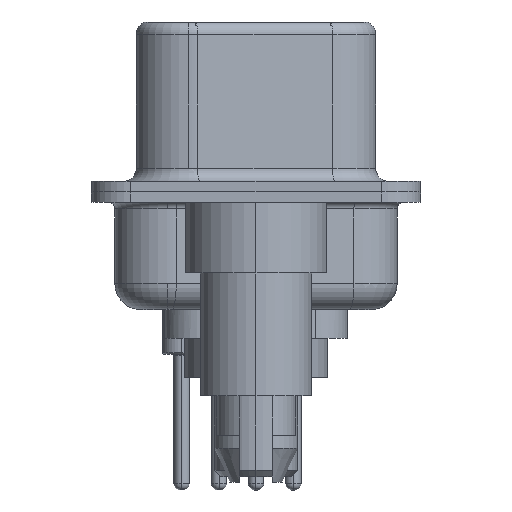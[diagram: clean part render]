
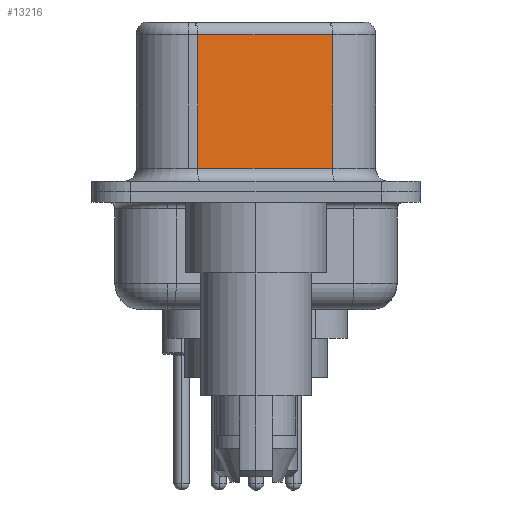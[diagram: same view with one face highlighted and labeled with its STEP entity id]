
A CAD part, left-side view. The second image highlights one B-rep face of the part: STEP entity #13216.
In plain terms, the highlighted planar face has unit normal (-0.985, -0.174, 0).
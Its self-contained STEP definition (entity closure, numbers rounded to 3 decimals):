
#67 = LINE ( 'NONE', #17907, #19690 ) ;
#342 = ORIENTED_EDGE ( 'NONE', *, *, #385, .T. ) ;
#385 = EDGE_CURVE ( 'NONE', #2215, #20481, #11124, .T. ) ;
#491 = EDGE_CURVE ( 'NONE', #8566, #9452, #790, .T. ) ;
#790 = LINE ( 'NONE', #3194, #10511 ) ;
#908 = CARTESIAN_POINT ( 'NONE',  ( 3.67, 2.233, 6.52 ) ) ;
#1786 = EDGE_CURVE ( 'NONE', #9452, #2215, #16957, .T. ) ;
#2215 = VERTEX_POINT ( 'NONE', #6479 ) ;
#3194 = CARTESIAN_POINT ( 'NONE',  ( 4.58, -2.927, 6.02 ) ) ;
#3202 = PLANE ( 'NONE',  #17059 ) ;
#3745 = EDGE_LOOP ( 'NONE', ( #22078, #18330, #22930, #342 ) ) ;
#4186 = FACE_OUTER_BOUND ( 'NONE', #3745, .T. ) ;
#4697 = DIRECTION ( 'NONE',  ( 0., 0., -1. ) ) ;
#5144 = DIRECTION ( 'NONE',  ( 0.985, 0.174, 0. ) ) ;
#5677 = CARTESIAN_POINT ( 'NONE',  ( 4.58, -2.927, 6.02 ) ) ;
#6188 = DIRECTION ( 'NONE',  ( 0., 0., -1. ) ) ;
#6479 = CARTESIAN_POINT ( 'NONE',  ( 3.67, 2.233, 0.9 ) ) ;
#8566 = VERTEX_POINT ( 'NONE', #5677 ) ;
#8741 = EDGE_CURVE ( 'NONE', #8566, #20481, #67, .T. ) ;
#9452 = VERTEX_POINT ( 'NONE', #18325 ) ;
#9867 = CARTESIAN_POINT ( 'NONE',  ( 4.58, -2.927, 0.9 ) ) ;
#10511 = VECTOR ( 'NONE', #16533, 1000. ) ;
#11124 = LINE ( 'NONE', #9867, #21603 ) ;
#11714 = VECTOR ( 'NONE', #4697, 1000. ) ;
#12050 = CARTESIAN_POINT ( 'NONE',  ( 4.58, -2.927, 0.9 ) ) ;
#13216 = ADVANCED_FACE ( 'NONE', ( #4186 ), #3202, .F. ) ;
#13439 = DIRECTION ( 'NONE',  ( 0.174, -0.985, 0. ) ) ;
#16533 = DIRECTION ( 'NONE',  ( -0.174, 0.985, 0. ) ) ;
#16957 = LINE ( 'NONE', #908, #11714 ) ;
#17059 = AXIS2_PLACEMENT_3D ( 'NONE', #22701, #5144, #18828 ) ;
#17907 = CARTESIAN_POINT ( 'NONE',  ( 4.58, -2.927, 6.52 ) ) ;
#18325 = CARTESIAN_POINT ( 'NONE',  ( 3.67, 2.233, 6.02 ) ) ;
#18330 = ORIENTED_EDGE ( 'NONE', *, *, #491, .T. ) ;
#18828 = DIRECTION ( 'NONE',  ( -0.174, 0.985, 0. ) ) ;
#19690 = VECTOR ( 'NONE', #6188, 1000. ) ;
#20481 = VERTEX_POINT ( 'NONE', #12050 ) ;
#21603 = VECTOR ( 'NONE', #13439, 1000. ) ;
#22078 = ORIENTED_EDGE ( 'NONE', *, *, #8741, .F. ) ;
#22701 = CARTESIAN_POINT ( 'NONE',  ( 4.58, -2.927, 6.52 ) ) ;
#22930 = ORIENTED_EDGE ( 'NONE', *, *, #1786, .T. ) ;
